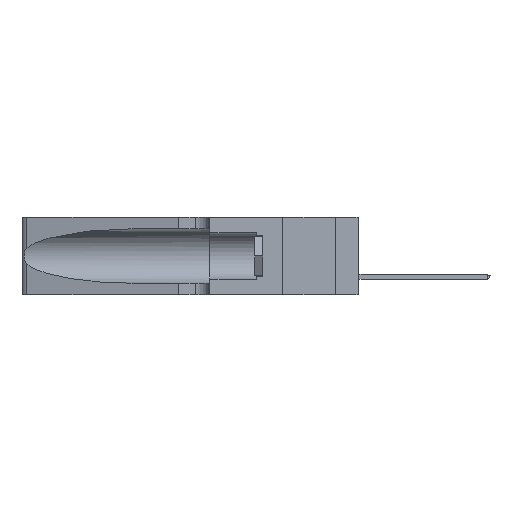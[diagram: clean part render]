
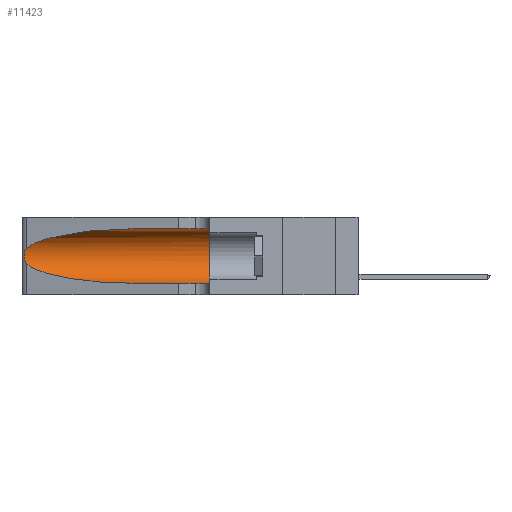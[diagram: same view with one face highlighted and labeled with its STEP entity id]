
A CAD part, left-side view. The second image highlights one B-rep face of the part: STEP entity #11423.
In plain terms, the highlighted cylindrical face has radius 3.308 mm (diameter 6.617 mm), a partial arc.
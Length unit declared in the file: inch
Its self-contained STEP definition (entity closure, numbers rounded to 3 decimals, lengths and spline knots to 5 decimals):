
#372 = CARTESIAN_POINT ( 'NONE',  ( 0.1305, 0.72297, 0.31525 ) ) ;
#482 = EDGE_CURVE ( 'NONE', #42351, #31125, #27354, .T. ) ;
#3775 = CARTESIAN_POINT ( 'NONE',  ( 0.25487, 1.22718, 0.22369 ) ) ;
#4468 = CARTESIAN_POINT ( 'NONE',  ( 0.1305, 0.72297, 0.05475 ) ) ;
#4483 = DIRECTION ( 'NONE',  ( 0., -1., 0. ) ) ;
#5020 = CARTESIAN_POINT ( 'NONE',  ( 0.25487, 1.22718, 0.22369 ) ) ;
#5139 = CARTESIAN_POINT ( 'NONE',  ( 0.25487, 1.22718, 0.22369 ) ) ;
#6402 = EDGE_CURVE ( 'NONE', #31125, #16955, #17824, .T. ) ;
#6600 = VERTEX_POINT ( 'NONE', #19902 ) ;
#6938 = ORIENTED_EDGE ( 'NONE', *, *, #37165, .T. ) ;
#8252 = CARTESIAN_POINT ( 'NONE',  ( 0.25487, 1.22718, 0.14631 ) ) ;
#8623 = FACE_OUTER_BOUND ( 'NONE', #10084, .T. ) ;
#8690 = CARTESIAN_POINT ( 'NONE',  ( 0.1305, 0.72297, 0.31525 ) ) ;
#10084 = EDGE_LOOP ( 'NONE', ( #19603, #6938, #12444, #43422, #37583, #43795 ) ) ;
#10135 = DIRECTION ( 'NONE',  ( 0., 0., -1. ) ) ;
#10229 =( BOUNDED_CURVE ( )  B_SPLINE_CURVE ( 3, ( #28026, #31119, #14394, #4468 ),
 .UNSPECIFIED., .F., .F. ) 
 B_SPLINE_CURVE_WITH_KNOTS ( ( 4, 4 ),
 ( 3.44316, 4.71239 ),
 .UNSPECIFIED. ) 
 CURVE ( )  GEOMETRIC_REPRESENTATION_ITEM ( )  RATIONAL_B_SPLINE_CURVE ( ( 1., 0.87, 0.87, 1. ) ) 
 REPRESENTATION_ITEM ( '' )  );
#11423 = ADVANCED_FACE ( 'NONE', ( #8623 ), #43615, .F. ) ;
#11675 = CARTESIAN_POINT ( 'NONE',  ( 0.25555, 1.22994, 0.2215 ) ) ;
#12444 = ORIENTED_EDGE ( 'NONE', *, *, #16893, .T. ) ;
#13907 = DIRECTION ( 'NONE',  ( 0., 0., 1. ) ) ;
#14394 = CARTESIAN_POINT ( 'NONE',  ( 0.18966, 0.96281, 0.05475 ) ) ;
#14809 = B_SPLINE_CURVE_WITH_KNOTS ( 'NONE', 3,
 ( #5020, #11675, #18819, #25020, #35247, #21585, #42511, #14903, #28740, #15229, #38975, #31650, #18513, #8252 ),
 .UNSPECIFIED., .F., .F.,
 ( 4, 2, 2, 2, 2, 2, 4 ),
 ( 0., 0.00027, 0.00053, 0.00107, 0.0016, 0.00187, 0.00214 ),
 .UNSPECIFIED. ) ;
#14903 = CARTESIAN_POINT ( 'NONE',  ( 0.26075, 1.23896, 0.178 ) ) ;
#15229 = CARTESIAN_POINT ( 'NONE',  ( 0.25856, 1.23593, 0.16098 ) ) ;
#16893 = EDGE_CURVE ( 'NONE', #34555, #6600, #10229, .T. ) ;
#16955 = VERTEX_POINT ( 'NONE', #21498 ) ;
#17824 = CIRCLE ( 'NONE', #34527, 0.13025 ) ;
#18113 =( BOUNDED_CURVE ( )  B_SPLINE_CURVE ( 3, ( #8690, #26086, #18644, #5139 ),
 .UNSPECIFIED., .F., .F. ) 
 B_SPLINE_CURVE_WITH_KNOTS ( ( 4, 4 ),
 ( 1.5708, 2.84003 ),
 .UNSPECIFIED. ) 
 CURVE ( )  GEOMETRIC_REPRESENTATION_ITEM ( )  RATIONAL_B_SPLINE_CURVE ( ( 1., 0.87, 0.87, 1. ) ) 
 REPRESENTATION_ITEM ( '' )  );
#18513 = CARTESIAN_POINT ( 'NONE',  ( 0.25555, 1.22993, 0.14849 ) ) ;
#18644 = CARTESIAN_POINT ( 'NONE',  ( 0.2373, 1.15595, 0.28018 ) ) ;
#18819 = CARTESIAN_POINT ( 'NONE',  ( 0.25639, 1.23184, 0.21858 ) ) ;
#19603 = ORIENTED_EDGE ( 'NONE', *, *, #31137, .T. ) ;
#19902 = CARTESIAN_POINT ( 'NONE',  ( 0.1305, 0.72297, 0.05475 ) ) ;
#21262 = CARTESIAN_POINT ( 'NONE',  ( 0.1305, 0.35, 0.31525 ) ) ;
#21498 = CARTESIAN_POINT ( 'NONE',  ( 0.1305, 0.35, 0.05475 ) ) ;
#21585 = CARTESIAN_POINT ( 'NONE',  ( 0.26018, 1.23835, 0.19895 ) ) ;
#22337 = DIRECTION ( 'NONE',  ( 0., -1., 0. ) ) ;
#22801 = CARTESIAN_POINT ( 'NONE',  ( 0.1305, 1.61858, 0.185 ) ) ;
#24367 = VERTEX_POINT ( 'NONE', #3775 ) ;
#25020 = CARTESIAN_POINT ( 'NONE',  ( 0.25787, 1.23484, 0.2124 ) ) ;
#25237 = VECTOR ( 'NONE', #4483, 39.37008 ) ;
#25542 = LINE ( 'NONE', #43472, #33482 ) ;
#26086 = CARTESIAN_POINT ( 'NONE',  ( 0.18966, 0.96281, 0.31525 ) ) ;
#27022 = DIRECTION ( 'NONE',  ( 0., 1., 0. ) ) ;
#27354 = LINE ( 'NONE', #38131, #25237 ) ;
#28026 = CARTESIAN_POINT ( 'NONE',  ( 0.25487, 1.22718, 0.14631 ) ) ;
#28677 = CARTESIAN_POINT ( 'NONE',  ( 0.25487, 1.22718, 0.14631 ) ) ;
#28740 = CARTESIAN_POINT ( 'NONE',  ( 0.26017, 1.23833, 0.17102 ) ) ;
#31119 = CARTESIAN_POINT ( 'NONE',  ( 0.2373, 1.15595, 0.08982 ) ) ;
#31125 = VERTEX_POINT ( 'NONE', #21262 ) ;
#31137 = EDGE_CURVE ( 'NONE', #42351, #24367, #18113, .T. ) ;
#31650 = CARTESIAN_POINT ( 'NONE',  ( 0.25639, 1.23186, 0.15144 ) ) ;
#33184 = EDGE_CURVE ( 'NONE', #6600, #16955, #25542, .T. ) ;
#33482 = VECTOR ( 'NONE', #41014, 39.37008 ) ;
#34527 = AXIS2_PLACEMENT_3D ( 'NONE', #37217, #27022, #13907 ) ;
#34555 = VERTEX_POINT ( 'NONE', #28677 ) ;
#35247 = CARTESIAN_POINT ( 'NONE',  ( 0.25854, 1.2359, 0.20912 ) ) ;
#37165 = EDGE_CURVE ( 'NONE', #24367, #34555, #14809, .T. ) ;
#37217 = CARTESIAN_POINT ( 'NONE',  ( 0.1305, 0.35, 0.185 ) ) ;
#37583 = ORIENTED_EDGE ( 'NONE', *, *, #6402, .F. ) ;
#38131 = CARTESIAN_POINT ( 'NONE',  ( 0.1305, 1.61858, 0.31525 ) ) ;
#38975 = CARTESIAN_POINT ( 'NONE',  ( 0.25789, 1.23486, 0.15765 ) ) ;
#41014 = DIRECTION ( 'NONE',  ( 0., -1., 0. ) ) ;
#41414 = AXIS2_PLACEMENT_3D ( 'NONE', #22801, #22337, #10135 ) ;
#42351 = VERTEX_POINT ( 'NONE', #372 ) ;
#42511 = CARTESIAN_POINT ( 'NONE',  ( 0.26075, 1.23896, 0.19203 ) ) ;
#43422 = ORIENTED_EDGE ( 'NONE', *, *, #33184, .T. ) ;
#43472 = CARTESIAN_POINT ( 'NONE',  ( 0.1305, 1.61858, 0.05475 ) ) ;
#43615 = CYLINDRICAL_SURFACE ( 'NONE', #41414, 0.13025 ) ;
#43795 = ORIENTED_EDGE ( 'NONE', *, *, #482, .F. ) ;
